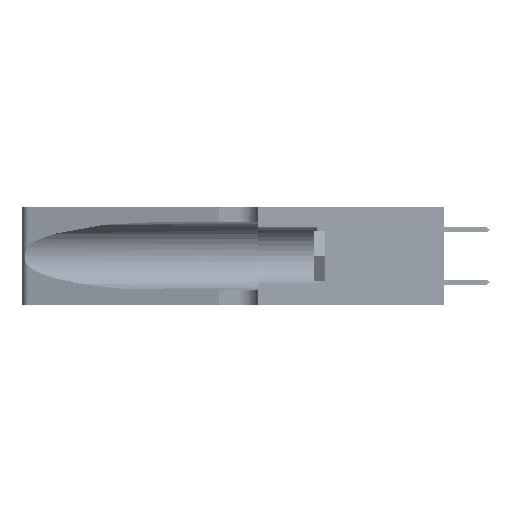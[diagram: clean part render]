
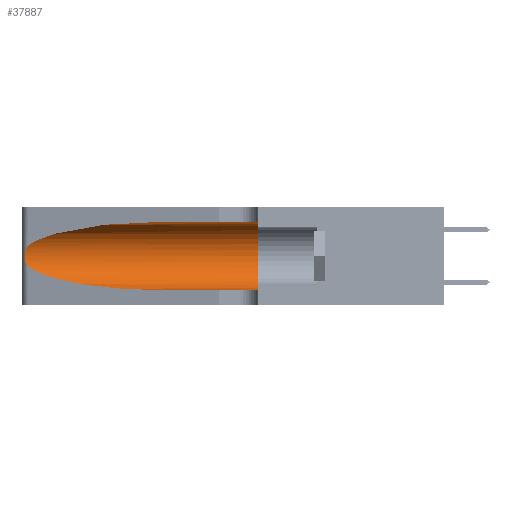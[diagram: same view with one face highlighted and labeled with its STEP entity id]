
A CAD part, left-side view. The second image highlights one B-rep face of the part: STEP entity #37887.
In plain terms, the highlighted cylindrical face has radius 3.308 mm (diameter 6.617 mm), a partial arc.
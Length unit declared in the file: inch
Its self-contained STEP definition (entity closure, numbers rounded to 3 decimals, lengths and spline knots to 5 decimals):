
#627 = VERTEX_POINT ( 'NONE', #48237 ) ;
#1337 = CARTESIAN_POINT ( 'NONE',  ( 0.1305, 0.35, 0.185 ) ) ;
#2135 = CARTESIAN_POINT ( 'NONE',  ( 0.26075, 1.23896, 0.178 ) ) ;
#3068 = VECTOR ( 'NONE', #25150, 39.37008 ) ;
#3133 = VERTEX_POINT ( 'NONE', #9163 ) ;
#3802 = DIRECTION ( 'NONE',  ( 0., -1., 0. ) ) ;
#4207 = CARTESIAN_POINT ( 'NONE',  ( 0.1305, 0.72297, 0.31525 ) ) ;
#4430 = ORIENTED_EDGE ( 'NONE', *, *, #7991, .T. ) ;
#5305 = CARTESIAN_POINT ( 'NONE',  ( 0.25787, 1.23484, 0.2124 ) ) ;
#5816 = CARTESIAN_POINT ( 'NONE',  ( 0.25854, 1.2359, 0.20912 ) ) ;
#7718 = ORIENTED_EDGE ( 'NONE', *, *, #21559, .F. ) ;
#7991 = EDGE_CURVE ( 'NONE', #627, #38300, #27236, .T. ) ;
#9163 = CARTESIAN_POINT ( 'NONE',  ( 0.1305, 0.35, 0.05475 ) ) ;
#9469 = CARTESIAN_POINT ( 'NONE',  ( 0.25555, 1.22993, 0.14849 ) ) ;
#11394 = ORIENTED_EDGE ( 'NONE', *, *, #12958, .T. ) ;
#12524 = ORIENTED_EDGE ( 'NONE', *, *, #44353, .F. ) ;
#12918 = CARTESIAN_POINT ( 'NONE',  ( 0.25487, 1.22718, 0.14631 ) ) ;
#12958 = EDGE_CURVE ( 'NONE', #38300, #36575, #21478, .T. ) ;
#13697 = LINE ( 'NONE', #33113, #3068 ) ;
#16538 = CARTESIAN_POINT ( 'NONE',  ( 0.25639, 1.23186, 0.15144 ) ) ;
#16877 = CARTESIAN_POINT ( 'NONE',  ( 0.26075, 1.23896, 0.19203 ) ) ;
#17215 = AXIS2_PLACEMENT_3D ( 'NONE', #1337, #46896, #20225 ) ;
#19660 = CARTESIAN_POINT ( 'NONE',  ( 0.2373, 1.15595, 0.08982 ) ) ;
#20225 = DIRECTION ( 'NONE',  ( 0., 0., 1. ) ) ;
#20907 = CARTESIAN_POINT ( 'NONE',  ( 0.1305, 0.35, 0.31525 ) ) ;
#21478 =( BOUNDED_CURVE ( )  B_SPLINE_CURVE ( 3, ( #30150, #19660, #31103, #38744 ),
 .UNSPECIFIED., .F., .T. ) 
 B_SPLINE_CURVE_WITH_KNOTS ( ( 4, 4 ),
 ( 3.44316, 4.71239 ),
 .UNSPECIFIED. ) 
 CURVE ( )  GEOMETRIC_REPRESENTATION_ITEM ( )  RATIONAL_B_SPLINE_CURVE ( ( 1., 0.87, 0.87, 1. ) ) 
 REPRESENTATION_ITEM ( '' )  );
#21559 = EDGE_CURVE ( 'NONE', #45427, #48093, #38153, .T. ) ;
#21582 = DIRECTION ( 'NONE',  ( 0., 0., -1. ) ) ;
#21963 = CARTESIAN_POINT ( 'NONE',  ( 0.25487, 1.22718, 0.22369 ) ) ;
#22116 = CARTESIAN_POINT ( 'NONE',  ( 0.2373, 1.15595, 0.28018 ) ) ;
#22418 = FACE_OUTER_BOUND ( 'NONE', #24317, .T. ) ;
#23575 = CARTESIAN_POINT ( 'NONE',  ( 0.1305, 0.72297, 0.31525 ) ) ;
#24185 = CARTESIAN_POINT ( 'NONE',  ( 0.1305, 1.61858, 0.31525 ) ) ;
#24317 = EDGE_LOOP ( 'NONE', ( #43658, #4430, #11394, #48444, #12524, #7718 ) ) ;
#24348 = CARTESIAN_POINT ( 'NONE',  ( 0.26017, 1.23833, 0.17102 ) ) ;
#24509 = CARTESIAN_POINT ( 'NONE',  ( 0.25856, 1.23593, 0.16098 ) ) ;
#24848 = CARTESIAN_POINT ( 'NONE',  ( 0.26018, 1.23835, 0.19895 ) ) ;
#25150 = DIRECTION ( 'NONE',  ( 0., -1., 0. ) ) ;
#27236 = B_SPLINE_CURVE_WITH_KNOTS ( 'NONE', 3,
 ( #32125, #39947, #28475, #5305, #5816, #24848, #16877, #2135, #24348, #24509, #28632, #16538, #9469, #12918 ),
 .UNSPECIFIED., .F., .F.,
 ( 4, 2, 2, 2, 2, 2, 4 ),
 ( 0., 0.00027, 0.00053, 0.00107, 0.0016, 0.00187, 0.00214 ),
 .UNSPECIFIED. ) ;
#27495 = VECTOR ( 'NONE', #3802, 39.37008 ) ;
#28475 = CARTESIAN_POINT ( 'NONE',  ( 0.25639, 1.23184, 0.21858 ) ) ;
#28632 = CARTESIAN_POINT ( 'NONE',  ( 0.25789, 1.23486, 0.15765 ) ) ;
#29200 = CARTESIAN_POINT ( 'NONE',  ( 0.1305, 1.61858, 0.185 ) ) ;
#29570 = CARTESIAN_POINT ( 'NONE',  ( 0.18966, 0.96281, 0.31525 ) ) ;
#29865 = DIRECTION ( 'NONE',  ( 0., -1., 0. ) ) ;
#30150 = CARTESIAN_POINT ( 'NONE',  ( 0.25487, 1.22718, 0.14631 ) ) ;
#31103 = CARTESIAN_POINT ( 'NONE',  ( 0.18966, 0.96281, 0.05475 ) ) ;
#32125 = CARTESIAN_POINT ( 'NONE',  ( 0.25487, 1.22718, 0.22369 ) ) ;
#33113 = CARTESIAN_POINT ( 'NONE',  ( 0.1305, 1.61858, 0.05475 ) ) ;
#35771 = CARTESIAN_POINT ( 'NONE',  ( 0.25487, 1.22718, 0.14631 ) ) ;
#36042 = EDGE_CURVE ( 'NONE', #36575, #3133, #13697, .T. ) ;
#36575 = VERTEX_POINT ( 'NONE', #36610 ) ;
#36610 = CARTESIAN_POINT ( 'NONE',  ( 0.1305, 0.72297, 0.05475 ) ) ;
#37887 = ADVANCED_FACE ( 'NONE', ( #22418 ), #44956, .F. ) ;
#38153 = LINE ( 'NONE', #24185, #27495 ) ;
#38300 = VERTEX_POINT ( 'NONE', #35771 ) ;
#38744 = CARTESIAN_POINT ( 'NONE',  ( 0.1305, 0.72297, 0.05475 ) ) ;
#39947 = CARTESIAN_POINT ( 'NONE',  ( 0.25555, 1.22994, 0.2215 ) ) ;
#42575 = CIRCLE ( 'NONE', #17215, 0.13025 ) ;
#43658 = ORIENTED_EDGE ( 'NONE', *, *, #45725, .T. ) ;
#44353 = EDGE_CURVE ( 'NONE', #48093, #3133, #42575, .T. ) ;
#44852 =( BOUNDED_CURVE ( )  B_SPLINE_CURVE ( 3, ( #23575, #29570, #22116, #21963 ),
 .UNSPECIFIED., .F., .F. ) 
 B_SPLINE_CURVE_WITH_KNOTS ( ( 4, 4 ),
 ( 1.5708, 2.84003 ),
 .UNSPECIFIED. ) 
 CURVE ( )  GEOMETRIC_REPRESENTATION_ITEM ( )  RATIONAL_B_SPLINE_CURVE ( ( 1., 0.87, 0.87, 1. ) ) 
 REPRESENTATION_ITEM ( '' )  );
#44956 = CYLINDRICAL_SURFACE ( 'NONE', #47188, 0.13025 ) ;
#45427 = VERTEX_POINT ( 'NONE', #4207 ) ;
#45725 = EDGE_CURVE ( 'NONE', #45427, #627, #44852, .T. ) ;
#46896 = DIRECTION ( 'NONE',  ( 0., 1., 0. ) ) ;
#47188 = AXIS2_PLACEMENT_3D ( 'NONE', #29200, #29865, #21582 ) ;
#48093 = VERTEX_POINT ( 'NONE', #20907 ) ;
#48237 = CARTESIAN_POINT ( 'NONE',  ( 0.25487, 1.22718, 0.22369 ) ) ;
#48444 = ORIENTED_EDGE ( 'NONE', *, *, #36042, .T. ) ;
